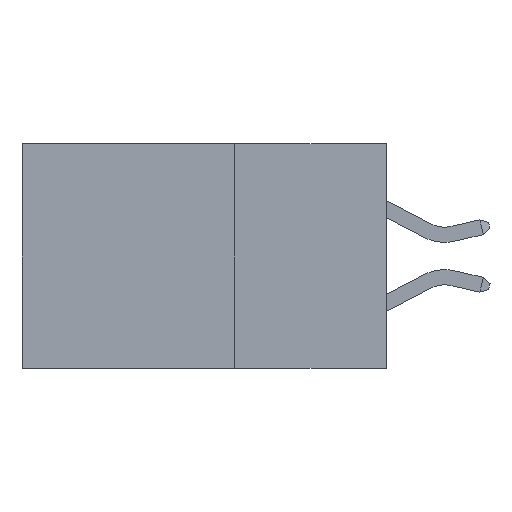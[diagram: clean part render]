
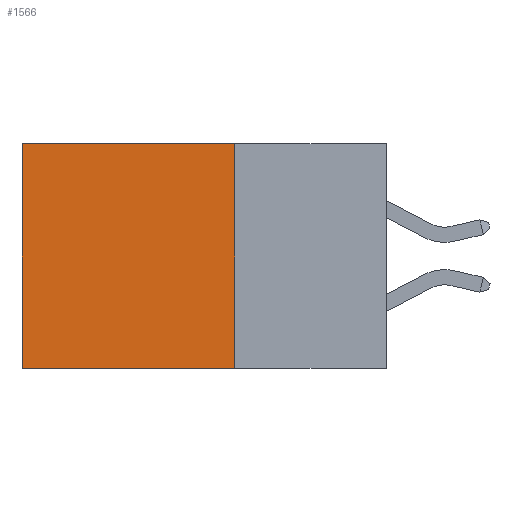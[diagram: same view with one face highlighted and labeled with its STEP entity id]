
A CAD part, left-side view. The second image highlights one B-rep face of the part: STEP entity #1566.
In plain terms, the highlighted planar face has unit normal (-1, 0, 0).
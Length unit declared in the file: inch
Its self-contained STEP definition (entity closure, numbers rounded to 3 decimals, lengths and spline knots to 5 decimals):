
#545 = LINE ( 'NONE', #9863, #11864 ) ;
#574 = DIRECTION ( 'NONE',  ( 0., 1., 0. ) ) ;
#733 = CARTESIAN_POINT ( 'NONE',  ( 0.2615, 0.25, -0.37 ) ) ;
#1405 = VECTOR ( 'NONE', #574, 39.37008 ) ;
#1477 = LINE ( 'NONE', #10267, #12606 ) ;
#1566 = ADVANCED_FACE ( 'NONE', ( #10694 ), #10311, .F. ) ;
#2238 = CARTESIAN_POINT ( 'NONE',  ( 0.2615, 0.25, 0. ) ) ;
#3390 = CARTESIAN_POINT ( 'NONE',  ( 0.2615, 0.6, 0. ) ) ;
#3496 = VERTEX_POINT ( 'NONE', #8835 ) ;
#5132 = EDGE_CURVE ( 'NONE', #12868, #13575, #1477, .T. ) ;
#6105 = ORIENTED_EDGE ( 'NONE', *, *, #12087, .F. ) ;
#6152 = EDGE_LOOP ( 'NONE', ( #11392, #6105, #9015, #11710 ) ) ;
#7008 = VECTOR ( 'NONE', #12895, 39.37008 ) ;
#7580 = EDGE_CURVE ( 'NONE', #10574, #3496, #545, .T. ) ;
#8326 = DIRECTION ( 'NONE',  ( 0., 0., -1. ) ) ;
#8835 = CARTESIAN_POINT ( 'NONE',  ( 0.2615, 0.25, -0.37 ) ) ;
#8916 = CARTESIAN_POINT ( 'NONE',  ( 0.2615, 0.25, 0. ) ) ;
#9015 = ORIENTED_EDGE ( 'NONE', *, *, #7580, .F. ) ;
#9769 = DIRECTION ( 'NONE',  ( 0., 0., -1. ) ) ;
#9848 = DIRECTION ( 'NONE',  ( 1., 0., 0. ) ) ;
#9863 = CARTESIAN_POINT ( 'NONE',  ( 0.2615, 0.25, -0.37 ) ) ;
#9877 = LINE ( 'NONE', #2238, #7008 ) ;
#10267 = CARTESIAN_POINT ( 'NONE',  ( 0.2615, 0.6, -0.37 ) ) ;
#10311 = PLANE ( 'NONE',  #11453 ) ;
#10574 = VERTEX_POINT ( 'NONE', #8916 ) ;
#10616 = DIRECTION ( 'NONE',  ( 0., 0., -1. ) ) ;
#10694 = FACE_OUTER_BOUND ( 'NONE', #6152, .T. ) ;
#10948 = CARTESIAN_POINT ( 'NONE',  ( 0.2615, 0.25, -0.37 ) ) ;
#11392 = ORIENTED_EDGE ( 'NONE', *, *, #5132, .T. ) ;
#11453 = AXIS2_PLACEMENT_3D ( 'NONE', #10948, #9848, #9769 ) ;
#11710 = ORIENTED_EDGE ( 'NONE', *, *, #13424, .T. ) ;
#11864 = VECTOR ( 'NONE', #8326, 39.37008 ) ;
#12087 = EDGE_CURVE ( 'NONE', #3496, #13575, #12543, .T. ) ;
#12310 = CARTESIAN_POINT ( 'NONE',  ( 0.2615, 0.6, -0.37 ) ) ;
#12543 = LINE ( 'NONE', #733, #1405 ) ;
#12606 = VECTOR ( 'NONE', #10616, 39.37008 ) ;
#12868 = VERTEX_POINT ( 'NONE', #3390 ) ;
#12895 = DIRECTION ( 'NONE',  ( 0., 1., 0. ) ) ;
#13424 = EDGE_CURVE ( 'NONE', #10574, #12868, #9877, .T. ) ;
#13575 = VERTEX_POINT ( 'NONE', #12310 ) ;
